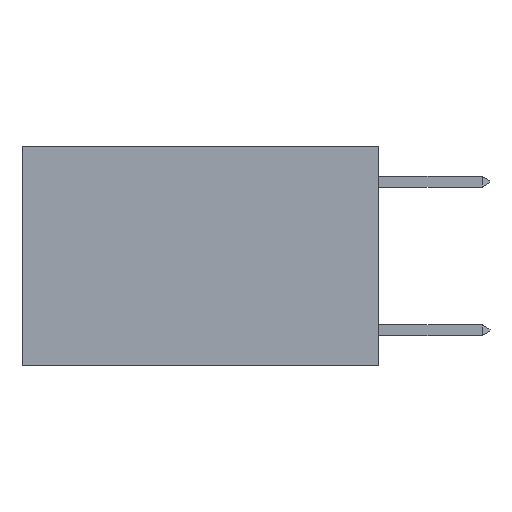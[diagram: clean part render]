
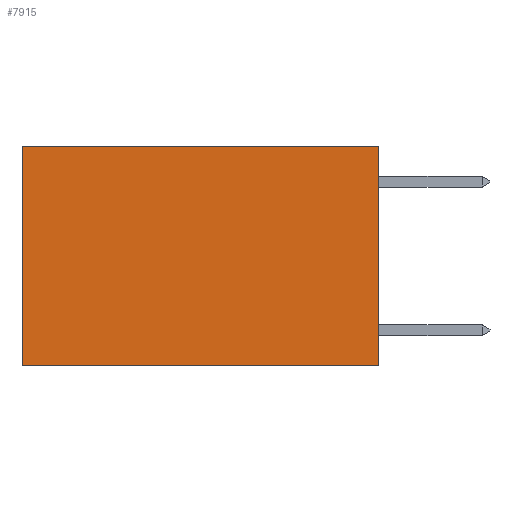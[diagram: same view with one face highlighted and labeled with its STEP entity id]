
A CAD part, left-side view. The second image highlights one B-rep face of the part: STEP entity #7915.
In plain terms, the highlighted planar face has unit normal (-1, 0, 0).
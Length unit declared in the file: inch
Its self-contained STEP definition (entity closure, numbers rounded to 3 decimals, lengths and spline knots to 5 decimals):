
#58 = VERTEX_POINT ( 'NONE', #4018 ) ;
#727 = ORIENTED_EDGE ( 'NONE', *, *, #5239, .F. ) ;
#1032 = ORIENTED_EDGE ( 'NONE', *, *, #6281, .F. ) ;
#1940 = LINE ( 'NONE', #7546, #6325 ) ;
#2253 = ORIENTED_EDGE ( 'NONE', *, *, #2917, .T. ) ;
#2460 = CARTESIAN_POINT ( 'NONE',  ( 0.2625, 0., 0. ) ) ;
#2578 = FACE_OUTER_BOUND ( 'NONE', #4989, .T. ) ;
#2592 = VECTOR ( 'NONE', #5769, 39.37008 ) ;
#2749 = CARTESIAN_POINT ( 'NONE',  ( 0.2625, 0., -0.37 ) ) ;
#2917 = EDGE_CURVE ( 'NONE', #7116, #58, #8491, .T. ) ;
#4009 = DIRECTION ( 'NONE',  ( 0., 0., -1. ) ) ;
#4018 = CARTESIAN_POINT ( 'NONE',  ( 0.2625, 0.6, 0. ) ) ;
#4250 = PLANE ( 'NONE',  #5964 ) ;
#4648 = VERTEX_POINT ( 'NONE', #2749 ) ;
#4989 = EDGE_LOOP ( 'NONE', ( #7152, #727, #1032, #2253 ) ) ;
#5048 = DIRECTION ( 'NONE',  ( 0., 0., -1. ) ) ;
#5049 = LINE ( 'NONE', #9948, #2592 ) ;
#5239 = EDGE_CURVE ( 'NONE', #4648, #7674, #5049, .T. ) ;
#5343 = CARTESIAN_POINT ( 'NONE',  ( 0.2625, 0., 0. ) ) ;
#5733 = CARTESIAN_POINT ( 'NONE',  ( 0.2625, 0.6, 0. ) ) ;
#5769 = DIRECTION ( 'NONE',  ( 0., 1., 0. ) ) ;
#5964 = AXIS2_PLACEMENT_3D ( 'NONE', #8442, #10078, #5048 ) ;
#6281 = EDGE_CURVE ( 'NONE', #7116, #4648, #1940, .T. ) ;
#6325 = VECTOR ( 'NONE', #7867, 39.37008 ) ;
#7086 = EDGE_CURVE ( 'NONE', #58, #7674, #7217, .T. ) ;
#7116 = VERTEX_POINT ( 'NONE', #2460 ) ;
#7152 = ORIENTED_EDGE ( 'NONE', *, *, #7086, .T. ) ;
#7217 = LINE ( 'NONE', #5733, #8011 ) ;
#7546 = CARTESIAN_POINT ( 'NONE',  ( 0.2625, 0., 0. ) ) ;
#7674 = VERTEX_POINT ( 'NONE', #9110 ) ;
#7867 = DIRECTION ( 'NONE',  ( 0., 0., -1. ) ) ;
#7915 = ADVANCED_FACE ( 'NONE', ( #2578 ), #4250, .F. ) ;
#8011 = VECTOR ( 'NONE', #4009, 39.37008 ) ;
#8442 = CARTESIAN_POINT ( 'NONE',  ( 0.2625, 0., 0. ) ) ;
#8491 = LINE ( 'NONE', #5343, #9903 ) ;
#9110 = CARTESIAN_POINT ( 'NONE',  ( 0.2625, 0.6, -0.37 ) ) ;
#9515 = DIRECTION ( 'NONE',  ( 0., 1., 0. ) ) ;
#9903 = VECTOR ( 'NONE', #9515, 39.37008 ) ;
#9948 = CARTESIAN_POINT ( 'NONE',  ( 0.2625, 0., -0.37 ) ) ;
#10078 = DIRECTION ( 'NONE',  ( 1., 0., 0. ) ) ;
